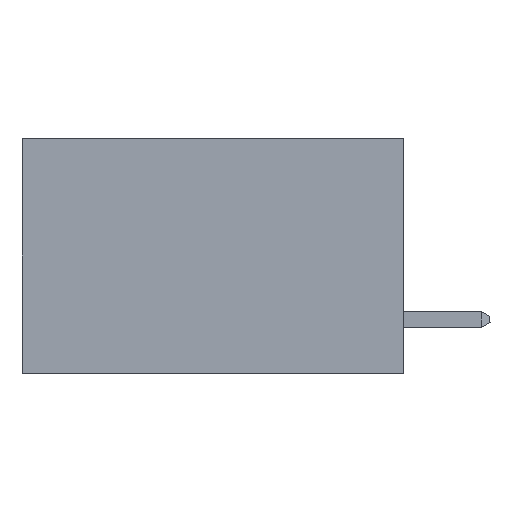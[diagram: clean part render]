
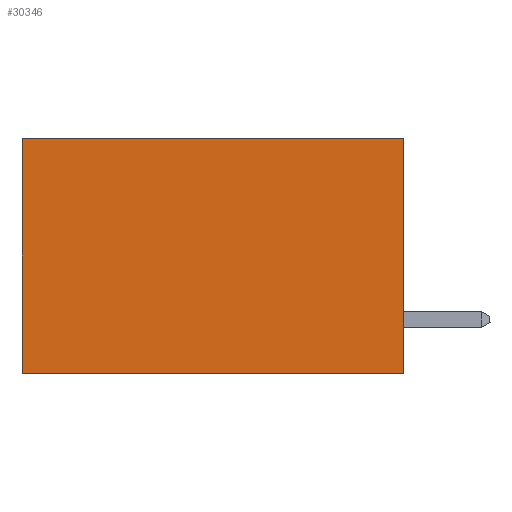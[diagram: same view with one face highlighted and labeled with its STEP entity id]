
A CAD part, left-side view. The second image highlights one B-rep face of the part: STEP entity #30346.
In plain terms, the highlighted planar face has unit normal (-1, 0, 0).
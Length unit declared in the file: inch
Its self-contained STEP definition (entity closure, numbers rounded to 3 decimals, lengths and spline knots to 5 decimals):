
#232 = VERTEX_POINT ( 'NONE', #818 ) ;
#818 = CARTESIAN_POINT ( 'NONE',  ( 0.2875, 0.6, -0.37 ) ) ;
#1632 = CARTESIAN_POINT ( 'NONE',  ( 0.2875, 0., -0.37 ) ) ;
#2803 = DIRECTION ( 'NONE',  ( 0., 1., 0. ) ) ;
#3295 = ORIENTED_EDGE ( 'NONE', *, *, #37399, .T. ) ;
#5901 = VECTOR ( 'NONE', #25427, 39.37008 ) ;
#7551 = AXIS2_PLACEMENT_3D ( 'NONE', #36748, #12923, #28187 ) ;
#8491 = ORIENTED_EDGE ( 'NONE', *, *, #27045, .F. ) ;
#8736 = CARTESIAN_POINT ( 'NONE',  ( 0.2875, 0., 0. ) ) ;
#9270 = VERTEX_POINT ( 'NONE', #18993 ) ;
#9436 = DIRECTION ( 'NONE',  ( 0., 0., -1. ) ) ;
#11231 = EDGE_CURVE ( 'NONE', #9270, #232, #21633, .T. ) ;
#12923 = DIRECTION ( 'NONE',  ( 1., 0., 0. ) ) ;
#15101 = LINE ( 'NONE', #1632, #39252 ) ;
#15169 = CARTESIAN_POINT ( 'NONE',  ( 0.2875, 0., 0. ) ) ;
#15567 = PLANE ( 'NONE',  #7551 ) ;
#16991 = EDGE_CURVE ( 'NONE', #24195, #22674, #39029, .T. ) ;
#17723 = ORIENTED_EDGE ( 'NONE', *, *, #11231, .T. ) ;
#18993 = CARTESIAN_POINT ( 'NONE',  ( 0.2875, 0.6, 0. ) ) ;
#19287 = CARTESIAN_POINT ( 'NONE',  ( 0.2875, 0.6, 0. ) ) ;
#19501 = EDGE_LOOP ( 'NONE', ( #17723, #8491, #23121, #3295 ) ) ;
#20723 = VECTOR ( 'NONE', #2803, 39.37008 ) ;
#21633 = LINE ( 'NONE', #19287, #5901 ) ;
#22674 = VERTEX_POINT ( 'NONE', #22811 ) ;
#22811 = CARTESIAN_POINT ( 'NONE',  ( 0.2875, 0., -0.37 ) ) ;
#23121 = ORIENTED_EDGE ( 'NONE', *, *, #16991, .F. ) ;
#24195 = VERTEX_POINT ( 'NONE', #15169 ) ;
#24917 = VECTOR ( 'NONE', #9436, 39.37008 ) ;
#25427 = DIRECTION ( 'NONE',  ( 0., 0., -1. ) ) ;
#25769 = FACE_OUTER_BOUND ( 'NONE', #19501, .T. ) ;
#27045 = EDGE_CURVE ( 'NONE', #22674, #232, #15101, .T. ) ;
#28187 = DIRECTION ( 'NONE',  ( 0., 0., -1. ) ) ;
#28807 = LINE ( 'NONE', #8736, #20723 ) ;
#29575 = DIRECTION ( 'NONE',  ( 0., 1., 0. ) ) ;
#30346 = ADVANCED_FACE ( 'NONE', ( #25769 ), #15567, .F. ) ;
#32626 = CARTESIAN_POINT ( 'NONE',  ( 0.2875, 0., 0. ) ) ;
#36748 = CARTESIAN_POINT ( 'NONE',  ( 0.2875, 0., 0. ) ) ;
#37399 = EDGE_CURVE ( 'NONE', #24195, #9270, #28807, .T. ) ;
#39029 = LINE ( 'NONE', #32626, #24917 ) ;
#39252 = VECTOR ( 'NONE', #29575, 39.37008 ) ;
